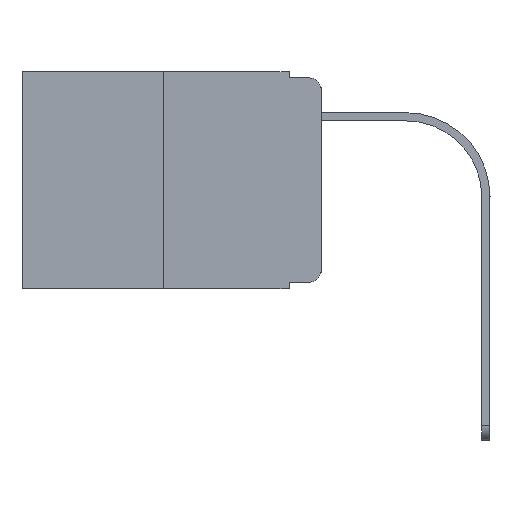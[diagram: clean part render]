
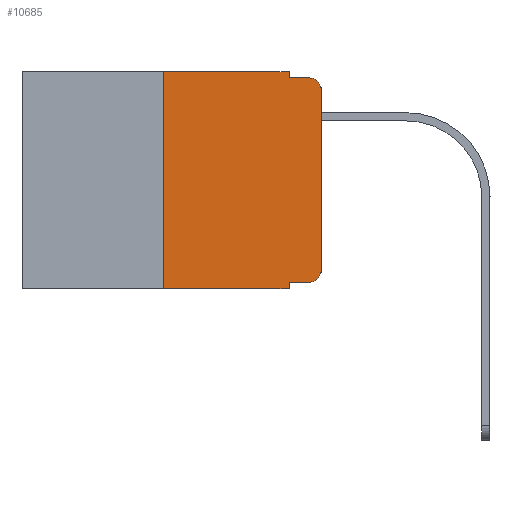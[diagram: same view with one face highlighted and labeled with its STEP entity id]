
A CAD part, left-side view. The second image highlights one B-rep face of the part: STEP entity #10685.
In plain terms, the highlighted planar face has unit normal (-1, 0, 0).
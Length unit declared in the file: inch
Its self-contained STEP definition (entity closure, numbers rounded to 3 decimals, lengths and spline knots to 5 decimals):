
#175 = LINE ( 'NONE', #6757, #6268 ) ;
#185 = DIRECTION ( 'NONE',  ( -1., 0., 0. ) ) ;
#213 = AXIS2_PLACEMENT_3D ( 'NONE', #13534, #895, #9435 ) ;
#223 = CARTESIAN_POINT ( 'NONE',  ( 0., 0.02, -0.333 ) ) ;
#228 = CARTESIAN_POINT ( 'NONE',  ( 0., 0.25, -0.343 ) ) ;
#250 = EDGE_CURVE ( 'NONE', #1982, #11654, #12280, .T. ) ;
#329 = DIRECTION ( 'NONE',  ( 0., 0., 1. ) ) ;
#345 = CARTESIAN_POINT ( 'NONE',  ( 0., 0.051, -0.333 ) ) ;
#471 = VECTOR ( 'NONE', #11870, 39.37008 ) ;
#895 = DIRECTION ( 'NONE',  ( -1., 0., 0. ) ) ;
#923 = CIRCLE ( 'NONE', #213, 0.02 ) ;
#1062 = ORIENTED_EDGE ( 'NONE', *, *, #11242, .T. ) ;
#1275 = DIRECTION ( 'NONE',  ( 1., 0., 0. ) ) ;
#1357 = VECTOR ( 'NONE', #5829, 39.37008 ) ;
#1371 = CARTESIAN_POINT ( 'NONE',  ( 0., 0.25, 0. ) ) ;
#1471 = VERTEX_POINT ( 'NONE', #13250 ) ;
#1982 = VERTEX_POINT ( 'NONE', #2696 ) ;
#2455 = VERTEX_POINT ( 'NONE', #5685 ) ;
#2469 = ORIENTED_EDGE ( 'NONE', *, *, #9188, .T. ) ;
#2674 = VERTEX_POINT ( 'NONE', #4270 ) ;
#2696 = CARTESIAN_POINT ( 'NONE',  ( 0., 0.051, -0.333 ) ) ;
#2711 = DIRECTION ( 'NONE',  ( 0., -1., 0. ) ) ;
#2762 = LINE ( 'NONE', #9331, #1357 ) ;
#3164 = VECTOR ( 'NONE', #4915, 39.37008 ) ;
#3267 = CARTESIAN_POINT ( 'NONE',  ( 0., 0.051, 0. ) ) ;
#3475 = EDGE_CURVE ( 'NONE', #11654, #2455, #923, .T. ) ;
#4001 = LINE ( 'NONE', #5197, #3164 ) ;
#4270 = CARTESIAN_POINT ( 'NONE',  ( 0., 0.02, -0.01 ) ) ;
#4457 = LINE ( 'NONE', #3267, #471 ) ;
#4493 = CARTESIAN_POINT ( 'NONE',  ( 0., 0.473, 0. ) ) ;
#4516 = EDGE_CURVE ( 'NONE', #1982, #1471, #4457, .T. ) ;
#4700 = AXIS2_PLACEMENT_3D ( 'NONE', #4493, #1275, #8909 ) ;
#4866 = ORIENTED_EDGE ( 'NONE', *, *, #5592, .F. ) ;
#4871 = EDGE_CURVE ( 'NONE', #11520, #2674, #6276, .T. ) ;
#4915 = DIRECTION ( 'NONE',  ( 0., 0., -1. ) ) ;
#4940 = AXIS2_PLACEMENT_3D ( 'NONE', #5486, #185, #7601 ) ;
#5043 = VECTOR ( 'NONE', #2711, 39.37008 ) ;
#5196 = VERTEX_POINT ( 'NONE', #10393 ) ;
#5197 = CARTESIAN_POINT ( 'NONE',  ( 0., 0.051, 0. ) ) ;
#5463 = FACE_OUTER_BOUND ( 'NONE', #7397, .T. ) ;
#5486 = CARTESIAN_POINT ( 'NONE',  ( 0., 0.02, -0.03 ) ) ;
#5592 = EDGE_CURVE ( 'NONE', #10776, #5196, #4001, .T. ) ;
#5685 = CARTESIAN_POINT ( 'NONE',  ( 0., 0., -0.313 ) ) ;
#5755 = CARTESIAN_POINT ( 'NONE',  ( 0., 0.25, 0. ) ) ;
#5829 = DIRECTION ( 'NONE',  ( 0., -1., 0. ) ) ;
#6124 = CARTESIAN_POINT ( 'NONE',  ( 0., 0.473, 0. ) ) ;
#6268 = VECTOR ( 'NONE', #6828, 39.37008 ) ;
#6276 = CIRCLE ( 'NONE', #4940, 0.02 ) ;
#6673 = VERTEX_POINT ( 'NONE', #5755 ) ;
#6757 = CARTESIAN_POINT ( 'NONE',  ( 0., 0.051, -0.01 ) ) ;
#6816 = CARTESIAN_POINT ( 'NONE',  ( 0., 0.051, 0. ) ) ;
#6828 = DIRECTION ( 'NONE',  ( 0., -1., 0. ) ) ;
#7051 = ORIENTED_EDGE ( 'NONE', *, *, #3475, .T. ) ;
#7397 = EDGE_LOOP ( 'NONE', ( #2469, #8866, #8763, #4866, #13112, #10972, #1062, #13091, #7426, #7051 ) ) ;
#7426 = ORIENTED_EDGE ( 'NONE', *, *, #250, .T. ) ;
#7601 = DIRECTION ( 'NONE',  ( 0., 0., -1. ) ) ;
#7643 = CARTESIAN_POINT ( 'NONE',  ( 0., 0., -0.03 ) ) ;
#7868 = PLANE ( 'NONE',  #4700 ) ;
#8049 = VECTOR ( 'NONE', #329, 39.37008 ) ;
#8070 = CARTESIAN_POINT ( 'NONE',  ( 0., 0., 0. ) ) ;
#8675 = VECTOR ( 'NONE', #12316, 39.37008 ) ;
#8763 = ORIENTED_EDGE ( 'NONE', *, *, #11145, .F. ) ;
#8866 = ORIENTED_EDGE ( 'NONE', *, *, #4871, .T. ) ;
#8909 = DIRECTION ( 'NONE',  ( 0., 0., -1. ) ) ;
#9188 = EDGE_CURVE ( 'NONE', #2455, #11520, #10163, .T. ) ;
#9331 = CARTESIAN_POINT ( 'NONE',  ( 0., 0.473, -0.343 ) ) ;
#9435 = DIRECTION ( 'NONE',  ( 0., 0., -1. ) ) ;
#9974 = LINE ( 'NONE', #1371, #8049 ) ;
#10163 = LINE ( 'NONE', #8070, #8675 ) ;
#10393 = CARTESIAN_POINT ( 'NONE',  ( 0., 0.051, -0.01 ) ) ;
#10412 = EDGE_CURVE ( 'NONE', #10811, #6673, #9974, .T. ) ;
#10488 = EDGE_CURVE ( 'NONE', #6673, #10776, #12462, .T. ) ;
#10685 = ADVANCED_FACE ( 'NONE', ( #5463 ), #7868, .F. ) ;
#10776 = VERTEX_POINT ( 'NONE', #6816 ) ;
#10811 = VERTEX_POINT ( 'NONE', #228 ) ;
#10972 = ORIENTED_EDGE ( 'NONE', *, *, #10412, .F. ) ;
#11145 = EDGE_CURVE ( 'NONE', #5196, #2674, #175, .T. ) ;
#11242 = EDGE_CURVE ( 'NONE', #10811, #1471, #2762, .T. ) ;
#11377 = VECTOR ( 'NONE', #12541, 39.37008 ) ;
#11520 = VERTEX_POINT ( 'NONE', #7643 ) ;
#11654 = VERTEX_POINT ( 'NONE', #223 ) ;
#11870 = DIRECTION ( 'NONE',  ( 0., 0., -1. ) ) ;
#12280 = LINE ( 'NONE', #345, #5043 ) ;
#12316 = DIRECTION ( 'NONE',  ( 0., 0., 1. ) ) ;
#12462 = LINE ( 'NONE', #6124, #11377 ) ;
#12541 = DIRECTION ( 'NONE',  ( 0., -1., 0. ) ) ;
#13091 = ORIENTED_EDGE ( 'NONE', *, *, #4516, .F. ) ;
#13112 = ORIENTED_EDGE ( 'NONE', *, *, #10488, .F. ) ;
#13250 = CARTESIAN_POINT ( 'NONE',  ( 0., 0.051, -0.343 ) ) ;
#13534 = CARTESIAN_POINT ( 'NONE',  ( 0., 0.02, -0.313 ) ) ;
